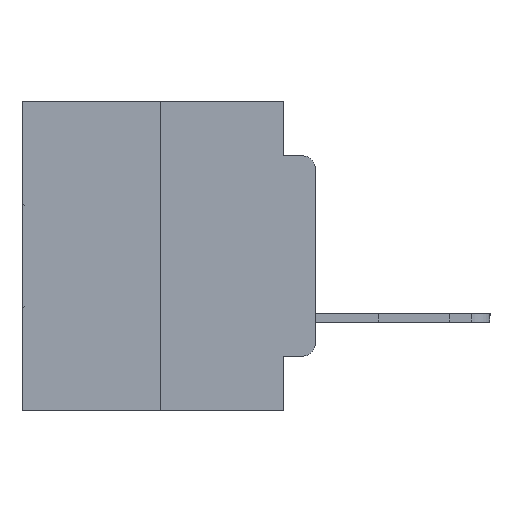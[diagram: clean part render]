
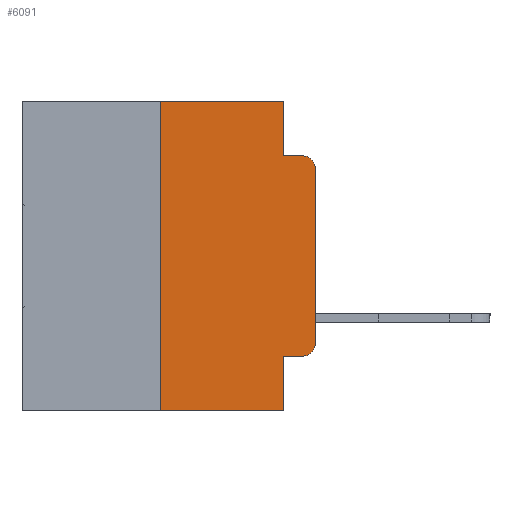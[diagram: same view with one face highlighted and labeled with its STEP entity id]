
A CAD part, left-side view. The second image highlights one B-rep face of the part: STEP entity #6091.
In plain terms, the highlighted planar face has unit normal (-1, 0, 0).
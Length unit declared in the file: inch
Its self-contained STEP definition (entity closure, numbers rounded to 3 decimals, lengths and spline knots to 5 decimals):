
#404 = LINE ( 'NONE', #25606, #18221 ) ;
#416 = ORIENTED_EDGE ( 'NONE', *, *, #2286, .T. ) ;
#441 = DIRECTION ( 'NONE',  ( -1., 0., 0. ) ) ;
#442 = VERTEX_POINT ( 'NONE', #27187 ) ;
#637 = VERTEX_POINT ( 'NONE', #20956 ) ;
#2286 = EDGE_CURVE ( 'NONE', #16274, #442, #19127, .T. ) ;
#2650 = EDGE_CURVE ( 'NONE', #3498, #14950, #16722, .T. ) ;
#2963 = EDGE_CURVE ( 'NONE', #12137, #8210, #15011, .T. ) ;
#3022 = CIRCLE ( 'NONE', #10676, 0.02 ) ;
#3124 = CARTESIAN_POINT ( 'NONE',  ( 0., 0., 0. ) ) ;
#3498 = VERTEX_POINT ( 'NONE', #27186 ) ;
#3739 = VECTOR ( 'NONE', #17649, 39.37008 ) ;
#4206 = AXIS2_PLACEMENT_3D ( 'NONE', #26348, #6591, #22058 ) ;
#5032 = ORIENTED_EDGE ( 'NONE', *, *, #12101, .T. ) ;
#5623 = DIRECTION ( 'NONE',  ( 0., -1., 0. ) ) ;
#6091 = ADVANCED_FACE ( 'NONE', ( #11407 ), #13292, .F. ) ;
#6129 = VECTOR ( 'NONE', #5623, 39.37008 ) ;
#6591 = DIRECTION ( 'NONE',  ( 1., 0., 0. ) ) ;
#6767 = ORIENTED_EDGE ( 'NONE', *, *, #2650, .F. ) ;
#7367 = DIRECTION ( 'NONE',  ( 0., 0., 1. ) ) ;
#7641 = CARTESIAN_POINT ( 'NONE',  ( 0., 0.051, -0.0885 ) ) ;
#7701 = CARTESIAN_POINT ( 'NONE',  ( 0., 0., -0.3915 ) ) ;
#8210 = VERTEX_POINT ( 'NONE', #20449 ) ;
#8447 = DIRECTION ( 'NONE',  ( 0., 0., 1. ) ) ;
#9918 = DIRECTION ( 'NONE',  ( 0., -1., 0. ) ) ;
#10005 = CARTESIAN_POINT ( 'NONE',  ( 0., 0.051, -0.4115 ) ) ;
#10328 = VECTOR ( 'NONE', #9918, 39.37008 ) ;
#10676 = AXIS2_PLACEMENT_3D ( 'NONE', #26479, #13438, #28649 ) ;
#11047 = LINE ( 'NONE', #23066, #16216 ) ;
#11407 = FACE_OUTER_BOUND ( 'NONE', #12346, .T. ) ;
#12086 = ORIENTED_EDGE ( 'NONE', *, *, #20170, .F. ) ;
#12101 = EDGE_CURVE ( 'NONE', #3498, #8210, #11047, .T. ) ;
#12137 = VERTEX_POINT ( 'NONE', #10005 ) ;
#12156 = LINE ( 'NONE', #18926, #6129 ) ;
#12346 = EDGE_LOOP ( 'NONE', ( #416, #20283, #21656, #27432, #12086, #6767, #5032, #16886, #12440, #24060 ) ) ;
#12440 = ORIENTED_EDGE ( 'NONE', *, *, #19004, .T. ) ;
#12536 = DIRECTION ( 'NONE',  ( 0., 0., -1. ) ) ;
#13292 = PLANE ( 'NONE',  #4206 ) ;
#13313 = VECTOR ( 'NONE', #7367, 39.37008 ) ;
#13438 = DIRECTION ( 'NONE',  ( -1., 0., 0. ) ) ;
#13922 = CARTESIAN_POINT ( 'NONE',  ( 0., 0.02, -0.1085 ) ) ;
#14228 = CARTESIAN_POINT ( 'NONE',  ( 0., 0.02, -0.0885 ) ) ;
#14323 = VECTOR ( 'NONE', #23865, 39.37008 ) ;
#14397 = CARTESIAN_POINT ( 'NONE',  ( 0., 0.473, 0. ) ) ;
#14403 = VERTEX_POINT ( 'NONE', #22251 ) ;
#14950 = VERTEX_POINT ( 'NONE', #18172 ) ;
#15011 = LINE ( 'NONE', #19277, #14323 ) ;
#15456 = CARTESIAN_POINT ( 'NONE',  ( 0., 0.051, -0.0885 ) ) ;
#16038 = VECTOR ( 'NONE', #8447, 39.37008 ) ;
#16128 = DIRECTION ( 'NONE',  ( 0., 0., -1. ) ) ;
#16216 = VECTOR ( 'NONE', #16470, 39.37008 ) ;
#16274 = VERTEX_POINT ( 'NONE', #7701 ) ;
#16470 = DIRECTION ( 'NONE',  ( 0., -1., 0. ) ) ;
#16722 = LINE ( 'NONE', #24774, #16038 ) ;
#16886 = ORIENTED_EDGE ( 'NONE', *, *, #2963, .F. ) ;
#17495 = VERTEX_POINT ( 'NONE', #14228 ) ;
#17649 = DIRECTION ( 'NONE',  ( 0., -1., 0. ) ) ;
#18001 = EDGE_CURVE ( 'NONE', #28347, #17495, #21448, .T. ) ;
#18073 = EDGE_CURVE ( 'NONE', #637, #16274, #3022, .T. ) ;
#18172 = CARTESIAN_POINT ( 'NONE',  ( 0., 0.25, 0. ) ) ;
#18221 = VECTOR ( 'NONE', #12536, 39.37008 ) ;
#18926 = CARTESIAN_POINT ( 'NONE',  ( 0., 0.051, -0.4115 ) ) ;
#19004 = EDGE_CURVE ( 'NONE', #12137, #637, #12156, .T. ) ;
#19127 = LINE ( 'NONE', #3124, #13313 ) ;
#19277 = CARTESIAN_POINT ( 'NONE',  ( 0., 0.051, 0. ) ) ;
#20170 = EDGE_CURVE ( 'NONE', #14950, #14403, #27098, .T. ) ;
#20283 = ORIENTED_EDGE ( 'NONE', *, *, #21851, .T. ) ;
#20449 = CARTESIAN_POINT ( 'NONE',  ( 0., 0.051, -0.5 ) ) ;
#20956 = CARTESIAN_POINT ( 'NONE',  ( 0., 0.02, -0.4115 ) ) ;
#21448 = LINE ( 'NONE', #15456, #3739 ) ;
#21656 = ORIENTED_EDGE ( 'NONE', *, *, #18001, .F. ) ;
#21851 = EDGE_CURVE ( 'NONE', #442, #17495, #23519, .T. ) ;
#22058 = DIRECTION ( 'NONE',  ( 0., 0., -1. ) ) ;
#22251 = CARTESIAN_POINT ( 'NONE',  ( 0., 0.051, 0. ) ) ;
#22696 = AXIS2_PLACEMENT_3D ( 'NONE', #13922, #441, #16128 ) ;
#23066 = CARTESIAN_POINT ( 'NONE',  ( 0., 0.473, -0.5 ) ) ;
#23519 = CIRCLE ( 'NONE', #22696, 0.02 ) ;
#23865 = DIRECTION ( 'NONE',  ( 0., 0., -1. ) ) ;
#24060 = ORIENTED_EDGE ( 'NONE', *, *, #18073, .T. ) ;
#24387 = EDGE_CURVE ( 'NONE', #14403, #28347, #404, .T. ) ;
#24774 = CARTESIAN_POINT ( 'NONE',  ( 0., 0.25, 0. ) ) ;
#25606 = CARTESIAN_POINT ( 'NONE',  ( 0., 0.051, 0. ) ) ;
#26348 = CARTESIAN_POINT ( 'NONE',  ( 0., 0.473, 0. ) ) ;
#26479 = CARTESIAN_POINT ( 'NONE',  ( 0., 0.02, -0.3915 ) ) ;
#27098 = LINE ( 'NONE', #14397, #10328 ) ;
#27186 = CARTESIAN_POINT ( 'NONE',  ( 0., 0.25, -0.5 ) ) ;
#27187 = CARTESIAN_POINT ( 'NONE',  ( 0., 0., -0.1085 ) ) ;
#27432 = ORIENTED_EDGE ( 'NONE', *, *, #24387, .F. ) ;
#28347 = VERTEX_POINT ( 'NONE', #7641 ) ;
#28649 = DIRECTION ( 'NONE',  ( 0., 0., -1. ) ) ;
